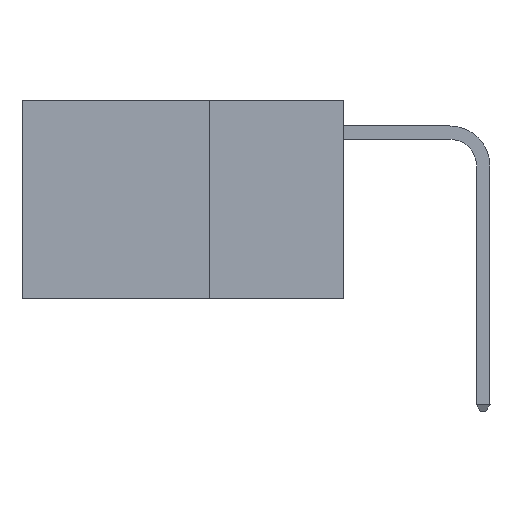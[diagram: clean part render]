
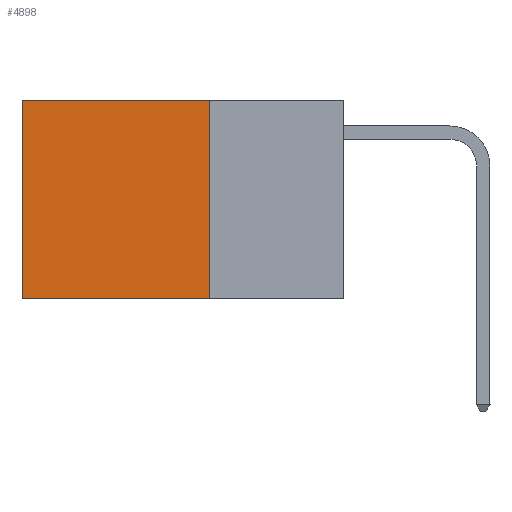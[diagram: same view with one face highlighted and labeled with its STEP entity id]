
A CAD part, left-side view. The second image highlights one B-rep face of the part: STEP entity #4898.
In plain terms, the highlighted planar face has unit normal (-1, 0, 0).
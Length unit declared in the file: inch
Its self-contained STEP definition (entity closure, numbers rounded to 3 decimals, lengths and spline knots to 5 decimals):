
#287 = LINE ( 'NONE', #9135, #13949 ) ;
#754 = CARTESIAN_POINT ( 'NONE',  ( 0.2625, 0.25, -0.37 ) ) ;
#1009 = EDGE_CURVE ( 'NONE', #2145, #3394, #12044, .T. ) ;
#1573 = VECTOR ( 'NONE', #10000, 39.37008 ) ;
#2145 = VERTEX_POINT ( 'NONE', #7209 ) ;
#2319 = LINE ( 'NONE', #14270, #11901 ) ;
#2621 = VECTOR ( 'NONE', #7501, 39.37008 ) ;
#3394 = VERTEX_POINT ( 'NONE', #754 ) ;
#3610 = CARTESIAN_POINT ( 'NONE',  ( 0.2625, 0.6, 0. ) ) ;
#4898 = ADVANCED_FACE ( 'NONE', ( #7838 ), #10503, .F. ) ;
#5181 = DIRECTION ( 'NONE',  ( 0., 1., 0. ) ) ;
#5963 = VERTEX_POINT ( 'NONE', #6036 ) ;
#6036 = CARTESIAN_POINT ( 'NONE',  ( 0.2625, 0.6, -0.37 ) ) ;
#7209 = CARTESIAN_POINT ( 'NONE',  ( 0.2625, 0.25, 0. ) ) ;
#7413 = EDGE_LOOP ( 'NONE', ( #12588, #12650, #12707, #12872 ) ) ;
#7501 = DIRECTION ( 'NONE',  ( 0., 0., -1. ) ) ;
#7838 = FACE_OUTER_BOUND ( 'NONE', #7413, .T. ) ;
#8195 = DIRECTION ( 'NONE',  ( 1., 0., 0. ) ) ;
#9135 = CARTESIAN_POINT ( 'NONE',  ( 0.2625, 0.25, 0. ) ) ;
#9553 = LINE ( 'NONE', #3610, #2621 ) ;
#9885 = CARTESIAN_POINT ( 'NONE',  ( 0.2625, 0.25, 0. ) ) ;
#10000 = DIRECTION ( 'NONE',  ( 0., 0., -1. ) ) ;
#10434 = DIRECTION ( 'NONE',  ( 0., 1., 0. ) ) ;
#10503 = PLANE ( 'NONE',  #12343 ) ;
#10562 = DIRECTION ( 'NONE',  ( 0., 0., -1. ) ) ;
#11504 = VERTEX_POINT ( 'NONE', #14388 ) ;
#11677 = CARTESIAN_POINT ( 'NONE',  ( 0.2625, 0.25, 0. ) ) ;
#11901 = VECTOR ( 'NONE', #5181, 39.37008 ) ;
#12044 = LINE ( 'NONE', #9885, #1573 ) ;
#12343 = AXIS2_PLACEMENT_3D ( 'NONE', #11677, #8195, #10562 ) ;
#12588 = ORIENTED_EDGE ( 'NONE', *, *, #12610, .T. ) ;
#12610 = EDGE_CURVE ( 'NONE', #11504, #5963, #9553, .T. ) ;
#12650 = ORIENTED_EDGE ( 'NONE', *, *, #15652, .F. ) ;
#12707 = ORIENTED_EDGE ( 'NONE', *, *, #1009, .F. ) ;
#12872 = ORIENTED_EDGE ( 'NONE', *, *, #14915, .T. ) ;
#13949 = VECTOR ( 'NONE', #10434, 39.37008 ) ;
#14270 = CARTESIAN_POINT ( 'NONE',  ( 0.2625, 0.25, -0.37 ) ) ;
#14388 = CARTESIAN_POINT ( 'NONE',  ( 0.2625, 0.6, 0. ) ) ;
#14915 = EDGE_CURVE ( 'NONE', #2145, #11504, #287, .T. ) ;
#15652 = EDGE_CURVE ( 'NONE', #3394, #5963, #2319, .T. ) ;
